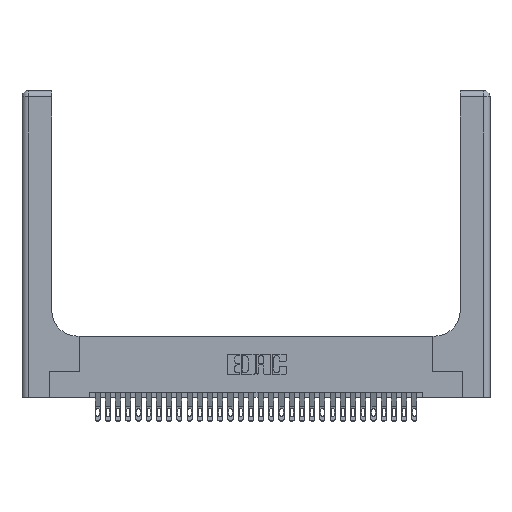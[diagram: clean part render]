
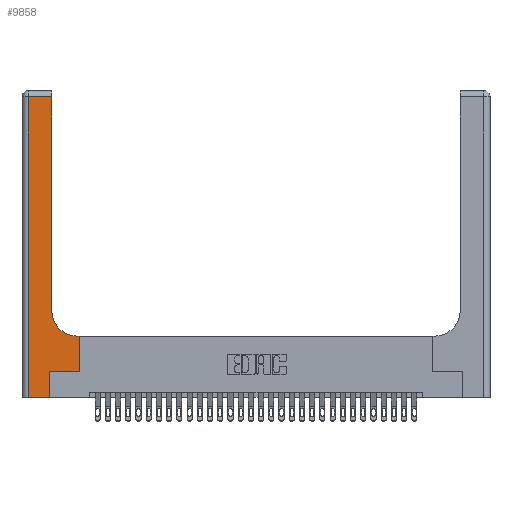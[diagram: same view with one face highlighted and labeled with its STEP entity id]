
A CAD part, top view. The second image highlights one B-rep face of the part: STEP entity #9858.
In plain terms, the highlighted planar face has unit normal (0, 0, 1).
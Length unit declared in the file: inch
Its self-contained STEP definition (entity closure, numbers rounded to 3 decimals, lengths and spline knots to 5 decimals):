
#173 = VERTEX_POINT ( 'NONE', #9288 ) ;
#237 = AXIS2_PLACEMENT_3D ( 'NONE', #17028, #27179, #7540 ) ;
#328 = VECTOR ( 'NONE', #10943, 39.37008 ) ;
#553 = VERTEX_POINT ( 'NONE', #15209 ) ;
#707 = ORIENTED_EDGE ( 'NONE', *, *, #7184, .T. ) ;
#902 = DIRECTION ( 'NONE',  ( -1., 0., 0. ) ) ;
#1010 = DIRECTION ( 'NONE',  ( 1., 0., 0. ) ) ;
#1459 = EDGE_CURVE ( 'NONE', #29423, #173, #20784, .T. ) ;
#1803 = CARTESIAN_POINT ( 'NONE',  ( 0.06, 2.94, 0.37 ) ) ;
#2535 = VECTOR ( 'NONE', #13783, 39.37008 ) ;
#2987 = CARTESIAN_POINT ( 'NONE',  ( 0.2915, 0.6, 0.37 ) ) ;
#3002 = DIRECTION ( 'NONE',  ( -1., 0., 0. ) ) ;
#3060 = LINE ( 'NONE', #26507, #328 ) ;
#3564 = DIRECTION ( 'NONE',  ( 1., 0., 0. ) ) ;
#4034 = EDGE_CURVE ( 'NONE', #5612, #6245, #29583, .T. ) ;
#4121 = CARTESIAN_POINT ( 'NONE',  ( 0.269, 0., 0.37 ) ) ;
#4519 = AXIS2_PLACEMENT_3D ( 'NONE', #5889, #10818, #1010 ) ;
#4755 = LINE ( 'NONE', #17728, #5154 ) ;
#5005 = ORIENTED_EDGE ( 'NONE', *, *, #4034, .T. ) ;
#5154 = VECTOR ( 'NONE', #3002, 39.37008 ) ;
#5256 = EDGE_CURVE ( 'NONE', #10181, #29423, #7071, .T. ) ;
#5434 = LINE ( 'NONE', #7660, #21930 ) ;
#5594 = CARTESIAN_POINT ( 'NONE',  ( 0.06, 0., 0.37 ) ) ;
#5612 = VERTEX_POINT ( 'NONE', #1803 ) ;
#5759 = CARTESIAN_POINT ( 'NONE',  ( 0.2915, 3., 0.37 ) ) ;
#5791 = VERTEX_POINT ( 'NONE', #30707 ) ;
#5874 = LINE ( 'NONE', #29903, #28248 ) ;
#5889 = CARTESIAN_POINT ( 'NONE',  ( 0.5415, 0.85, 0.37 ) ) ;
#6245 = VERTEX_POINT ( 'NONE', #5594 ) ;
#6678 = VERTEX_POINT ( 'NONE', #17482 ) ;
#6747 = ORIENTED_EDGE ( 'NONE', *, *, #25911, .T. ) ;
#6884 = FACE_OUTER_BOUND ( 'NONE', #12101, .T. ) ;
#7071 = CIRCLE ( 'NONE', #4519, 0.25 ) ;
#7184 = EDGE_CURVE ( 'NONE', #6245, #24707, #5874, .T. ) ;
#7540 = DIRECTION ( 'NONE',  ( -1., 0., 0. ) ) ;
#7660 = CARTESIAN_POINT ( 'NONE',  ( 0.5585, 0.25, 0.37 ) ) ;
#9288 = CARTESIAN_POINT ( 'NONE',  ( 0.2915, 2.94, 0.37 ) ) ;
#9415 = EDGE_CURVE ( 'NONE', #24707, #553, #3060, .T. ) ;
#9858 = ADVANCED_FACE ( 'NONE', ( #6884 ), #14968, .F. ) ;
#10181 = VERTEX_POINT ( 'NONE', #16602 ) ;
#10569 = EDGE_CURVE ( 'NONE', #553, #6678, #22602, .T. ) ;
#10818 = DIRECTION ( 'NONE',  ( 0., 0., -1. ) ) ;
#10943 = DIRECTION ( 'NONE',  ( 0., 1., 0. ) ) ;
#11255 = ORIENTED_EDGE ( 'NONE', *, *, #20374, .T. ) ;
#11272 = ORIENTED_EDGE ( 'NONE', *, *, #5256, .T. ) ;
#12101 = EDGE_LOOP ( 'NONE', ( #18980, #25812, #5005, #707, #29854, #15071, #11255, #6747, #11272 ) ) ;
#13570 = CARTESIAN_POINT ( 'NONE',  ( 0.269, 0.25, 0.37 ) ) ;
#13783 = DIRECTION ( 'NONE',  ( 0., -1., 0. ) ) ;
#14208 = VECTOR ( 'NONE', #22965, 39.37008 ) ;
#14683 = LINE ( 'NONE', #2987, #22763 ) ;
#14968 = PLANE ( 'NONE',  #237 ) ;
#15071 = ORIENTED_EDGE ( 'NONE', *, *, #10569, .T. ) ;
#15209 = CARTESIAN_POINT ( 'NONE',  ( 0.269, 0.25, 0.37 ) ) ;
#16602 = CARTESIAN_POINT ( 'NONE',  ( 0.5415, 0.6, 0.37 ) ) ;
#16721 = CARTESIAN_POINT ( 'NONE',  ( 0.2915, 0.85, 0.37 ) ) ;
#17028 = CARTESIAN_POINT ( 'NONE',  ( 0., 3., 0.37 ) ) ;
#17482 = CARTESIAN_POINT ( 'NONE',  ( 0.5585, 0.25, 0.37 ) ) ;
#17728 = CARTESIAN_POINT ( 'NONE',  ( 0., 2.94, 0.37 ) ) ;
#18980 = ORIENTED_EDGE ( 'NONE', *, *, #1459, .T. ) ;
#19965 = EDGE_CURVE ( 'NONE', #173, #5612, #4755, .T. ) ;
#20374 = EDGE_CURVE ( 'NONE', #6678, #5791, #5434, .T. ) ;
#20784 = LINE ( 'NONE', #5759, #14208 ) ;
#21930 = VECTOR ( 'NONE', #27306, 39.37008 ) ;
#22602 = LINE ( 'NONE', #13570, #30007 ) ;
#22763 = VECTOR ( 'NONE', #902, 39.37008 ) ;
#22902 = CARTESIAN_POINT ( 'NONE',  ( 0.06, 3., 0.37 ) ) ;
#22965 = DIRECTION ( 'NONE',  ( 0., 1., 0. ) ) ;
#24707 = VERTEX_POINT ( 'NONE', #4121 ) ;
#24966 = DIRECTION ( 'NONE',  ( 1., 0., 0. ) ) ;
#25812 = ORIENTED_EDGE ( 'NONE', *, *, #19965, .T. ) ;
#25911 = EDGE_CURVE ( 'NONE', #5791, #10181, #14683, .T. ) ;
#26507 = CARTESIAN_POINT ( 'NONE',  ( 0.269, 0., 0.37 ) ) ;
#27179 = DIRECTION ( 'NONE',  ( 0., 0., -1. ) ) ;
#27306 = DIRECTION ( 'NONE',  ( 0., 1., 0. ) ) ;
#28248 = VECTOR ( 'NONE', #24966, 39.37008 ) ;
#29423 = VERTEX_POINT ( 'NONE', #16721 ) ;
#29583 = LINE ( 'NONE', #22902, #2535 ) ;
#29854 = ORIENTED_EDGE ( 'NONE', *, *, #9415, .T. ) ;
#29903 = CARTESIAN_POINT ( 'NONE',  ( 0., 0., 0.37 ) ) ;
#30007 = VECTOR ( 'NONE', #3564, 39.37008 ) ;
#30707 = CARTESIAN_POINT ( 'NONE',  ( 0.5585, 0.6, 0.37 ) ) ;
